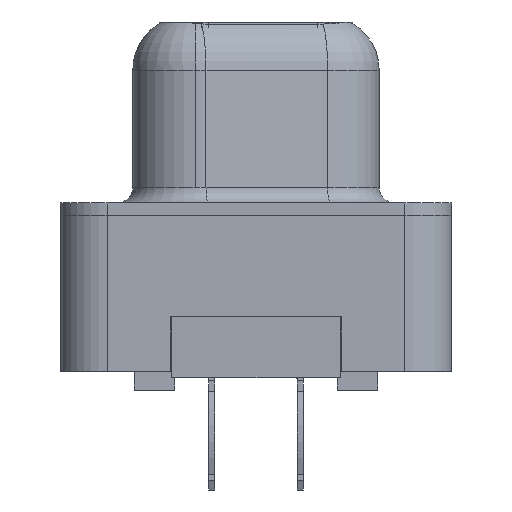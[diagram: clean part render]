
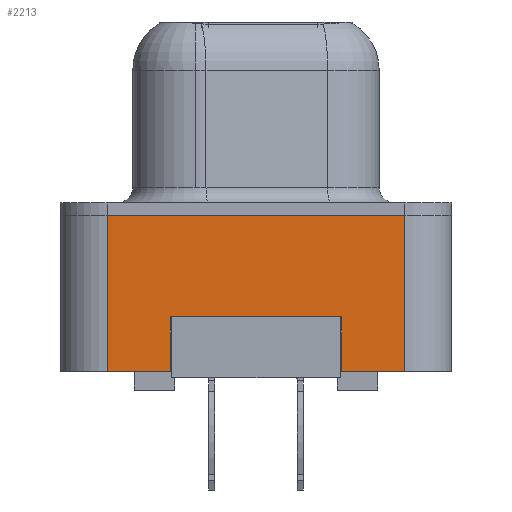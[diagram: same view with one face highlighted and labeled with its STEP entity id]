
A CAD part, left-side view. The second image highlights one B-rep face of the part: STEP entity #2213.
In plain terms, the highlighted planar face has unit normal (-1, 0, 0).
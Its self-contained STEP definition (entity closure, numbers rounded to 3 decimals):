
#357 = CARTESIAN_POINT ( 'NONE',  ( -2.945, 2.75, -3.25 ) ) ;
#610 = VERTEX_POINT ( 'NONE', #7063 ) ;
#670 = LINE ( 'NONE', #18458, #5891 ) ;
#1159 = LINE ( 'NONE', #4343, #9432 ) ;
#1741 = EDGE_CURVE ( 'NONE', #16292, #610, #1159, .T. ) ;
#1822 = LINE ( 'NONE', #7815, #9203 ) ;
#2213 = ADVANCED_FACE ( 'NONE', ( #14033 ), #2347, .T. ) ;
#2347 = PLANE ( 'NONE',  #3816 ) ;
#2373 = LINE ( 'NONE', #15808, #14583 ) ;
#2431 = ORIENTED_EDGE ( 'NONE', *, *, #9282, .F. ) ;
#3015 = EDGE_CURVE ( 'NONE', #4088, #8618, #7027, .T. ) ;
#3316 = DIRECTION ( 'NONE',  ( 0., -1., 0. ) ) ;
#3541 = DIRECTION ( 'NONE',  ( 0., 1., 0. ) ) ;
#3816 = AXIS2_PLACEMENT_3D ( 'NONE', #6811, #4277, #8717 ) ;
#3839 = ORIENTED_EDGE ( 'NONE', *, *, #10135, .F. ) ;
#3964 = CARTESIAN_POINT ( 'NONE',  ( -2.945, -4.775, -5. ) ) ;
#4088 = VERTEX_POINT ( 'NONE', #4551 ) ;
#4277 = DIRECTION ( 'NONE',  ( -1., 0., 0. ) ) ;
#4343 = CARTESIAN_POINT ( 'NONE',  ( -2.945, -4.775, -5. ) ) ;
#4547 = EDGE_CURVE ( 'NONE', #11308, #10992, #1822, .T. ) ;
#4551 = CARTESIAN_POINT ( 'NONE',  ( -2.945, -2.75, -3.25 ) ) ;
#4829 = LINE ( 'NONE', #10713, #9670 ) ;
#4862 = CARTESIAN_POINT ( 'NONE',  ( -2.945, 2.75, -3.25 ) ) ;
#5119 = ORIENTED_EDGE ( 'NONE', *, *, #1741, .T. ) ;
#5627 = DIRECTION ( 'NONE',  ( 0., 0., 1. ) ) ;
#5782 = CARTESIAN_POINT ( 'NONE',  ( -2.945, 4.775, 0. ) ) ;
#5891 = VECTOR ( 'NONE', #9550, 1000. ) ;
#6811 = CARTESIAN_POINT ( 'NONE',  ( -2.945, -4.775, -5. ) ) ;
#6899 = VECTOR ( 'NONE', #6927, 1000. ) ;
#6927 = DIRECTION ( 'NONE',  ( 0., 0., -1. ) ) ;
#7027 = LINE ( 'NONE', #17360, #6899 ) ;
#7063 = CARTESIAN_POINT ( 'NONE',  ( -2.945, -4.775, 0. ) ) ;
#7158 = EDGE_CURVE ( 'NONE', #8618, #16292, #13530, .T. ) ;
#7719 = LINE ( 'NONE', #357, #13550 ) ;
#7815 = CARTESIAN_POINT ( 'NONE',  ( -2.945, -4.775, -5. ) ) ;
#7972 = ORIENTED_EDGE ( 'NONE', *, *, #14402, .F. ) ;
#8288 = EDGE_LOOP ( 'NONE', ( #11174, #17946, #5119, #7972, #3839, #17558, #19023, #2431 ) ) ;
#8427 = EDGE_CURVE ( 'NONE', #18405, #10992, #2373, .T. ) ;
#8496 = VECTOR ( 'NONE', #3316, 1000. ) ;
#8618 = VERTEX_POINT ( 'NONE', #13772 ) ;
#8717 = DIRECTION ( 'NONE',  ( 0., 0., 1. ) ) ;
#9203 = VECTOR ( 'NONE', #10323, 1000. ) ;
#9282 = EDGE_CURVE ( 'NONE', #4088, #18405, #7719, .T. ) ;
#9432 = VECTOR ( 'NONE', #5627, 1000. ) ;
#9550 = DIRECTION ( 'NONE',  ( 0., 0., 1. ) ) ;
#9670 = VECTOR ( 'NONE', #11966, 1000. ) ;
#9985 = CARTESIAN_POINT ( 'NONE',  ( -2.945, 4.775, -5. ) ) ;
#10135 = EDGE_CURVE ( 'NONE', #11308, #13402, #670, .T. ) ;
#10323 = DIRECTION ( 'NONE',  ( 0., -1., 0. ) ) ;
#10713 = CARTESIAN_POINT ( 'NONE',  ( -2.945, -4.775, 0. ) ) ;
#10728 = CARTESIAN_POINT ( 'NONE',  ( -2.945, 2.75, -5. ) ) ;
#10992 = VERTEX_POINT ( 'NONE', #10728 ) ;
#11174 = ORIENTED_EDGE ( 'NONE', *, *, #3015, .T. ) ;
#11270 = DIRECTION ( 'NONE',  ( 0., 0., -1. ) ) ;
#11308 = VERTEX_POINT ( 'NONE', #9985 ) ;
#11966 = DIRECTION ( 'NONE',  ( 0., -1., 0. ) ) ;
#13402 = VERTEX_POINT ( 'NONE', #5782 ) ;
#13530 = LINE ( 'NONE', #18100, #8496 ) ;
#13550 = VECTOR ( 'NONE', #3541, 1000. ) ;
#13772 = CARTESIAN_POINT ( 'NONE',  ( -2.945, -2.75, -5. ) ) ;
#14033 = FACE_OUTER_BOUND ( 'NONE', #8288, .T. ) ;
#14402 = EDGE_CURVE ( 'NONE', #13402, #610, #4829, .T. ) ;
#14583 = VECTOR ( 'NONE', #11270, 1000. ) ;
#15808 = CARTESIAN_POINT ( 'NONE',  ( -2.945, 2.75, -3.25 ) ) ;
#16292 = VERTEX_POINT ( 'NONE', #3964 ) ;
#17360 = CARTESIAN_POINT ( 'NONE',  ( -2.945, -2.75, -3.25 ) ) ;
#17558 = ORIENTED_EDGE ( 'NONE', *, *, #4547, .T. ) ;
#17946 = ORIENTED_EDGE ( 'NONE', *, *, #7158, .T. ) ;
#18100 = CARTESIAN_POINT ( 'NONE',  ( -2.945, -4.775, -5. ) ) ;
#18405 = VERTEX_POINT ( 'NONE', #4862 ) ;
#18458 = CARTESIAN_POINT ( 'NONE',  ( -2.945, 4.775, -5. ) ) ;
#19023 = ORIENTED_EDGE ( 'NONE', *, *, #8427, .F. ) ;
